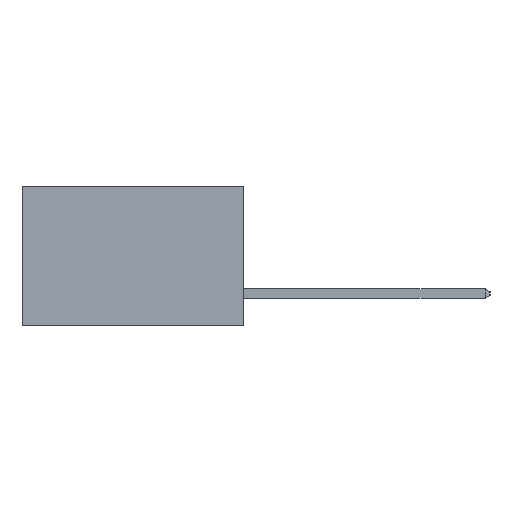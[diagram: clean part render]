
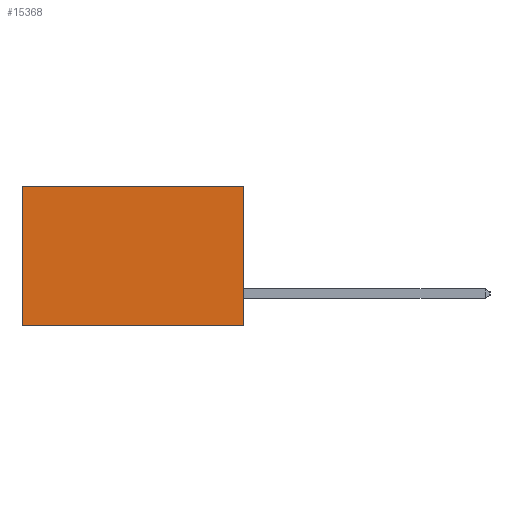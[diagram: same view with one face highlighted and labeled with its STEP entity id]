
A CAD part, left-side view. The second image highlights one B-rep face of the part: STEP entity #15368.
In plain terms, the highlighted planar face has unit normal (-1, 0, 0).
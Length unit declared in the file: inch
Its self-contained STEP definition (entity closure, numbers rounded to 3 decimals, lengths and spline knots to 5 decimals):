
#31 = VECTOR ( 'NONE', #7765, 39.37008 ) ;
#1726 = VECTOR ( 'NONE', #19805, 39.37008 ) ;
#2255 = VECTOR ( 'NONE', #12954, 39.37008 ) ;
#2284 = FACE_OUTER_BOUND ( 'NONE', #19009, .T. ) ;
#2792 = CARTESIAN_POINT ( 'NONE',  ( 0.277, 0.59, 0. ) ) ;
#2856 = EDGE_CURVE ( 'NONE', #18014, #8481, #8822, .T. ) ;
#4262 = LINE ( 'NONE', #10218, #20823 ) ;
#4377 = DIRECTION ( 'NONE',  ( 1., 0., 0. ) ) ;
#5814 = ORIENTED_EDGE ( 'NONE', *, *, #16967, .F. ) ;
#6081 = LINE ( 'NONE', #8632, #1726 ) ;
#7255 = CARTESIAN_POINT ( 'NONE',  ( 0.277, 0.59, -0.37 ) ) ;
#7581 = CARTESIAN_POINT ( 'NONE',  ( 0.277, 0., -0.37 ) ) ;
#7765 = DIRECTION ( 'NONE',  ( 0., 1., 0. ) ) ;
#8481 = VERTEX_POINT ( 'NONE', #7255 ) ;
#8632 = CARTESIAN_POINT ( 'NONE',  ( 0.277, 0., 0. ) ) ;
#8822 = LINE ( 'NONE', #17633, #31 ) ;
#9322 = VERTEX_POINT ( 'NONE', #2792 ) ;
#9854 = ORIENTED_EDGE ( 'NONE', *, *, #11756, .T. ) ;
#10218 = CARTESIAN_POINT ( 'NONE',  ( 0.277, 0., -0.37 ) ) ;
#11756 = EDGE_CURVE ( 'NONE', #9322, #8481, #15710, .T. ) ;
#12264 = AXIS2_PLACEMENT_3D ( 'NONE', #7581, #4377, #15701 ) ;
#12954 = DIRECTION ( 'NONE',  ( 0., 0., -1. ) ) ;
#13181 = CARTESIAN_POINT ( 'NONE',  ( 0.277, 0., -0.37 ) ) ;
#13471 = DIRECTION ( 'NONE',  ( 0., 0., -1. ) ) ;
#14090 = PLANE ( 'NONE',  #12264 ) ;
#14883 = VERTEX_POINT ( 'NONE', #19246 ) ;
#15368 = ADVANCED_FACE ( 'NONE', ( #2284 ), #14090, .F. ) ;
#15701 = DIRECTION ( 'NONE',  ( 0., 0., -1. ) ) ;
#15710 = LINE ( 'NONE', #20844, #2255 ) ;
#15923 = ORIENTED_EDGE ( 'NONE', *, *, #2856, .F. ) ;
#16291 = EDGE_CURVE ( 'NONE', #14883, #9322, #6081, .T. ) ;
#16967 = EDGE_CURVE ( 'NONE', #14883, #18014, #4262, .T. ) ;
#17633 = CARTESIAN_POINT ( 'NONE',  ( 0.277, 0., -0.37 ) ) ;
#18014 = VERTEX_POINT ( 'NONE', #13181 ) ;
#18469 = ORIENTED_EDGE ( 'NONE', *, *, #16291, .T. ) ;
#19009 = EDGE_LOOP ( 'NONE', ( #9854, #15923, #5814, #18469 ) ) ;
#19246 = CARTESIAN_POINT ( 'NONE',  ( 0.277, 0., 0. ) ) ;
#19805 = DIRECTION ( 'NONE',  ( 0., 1., 0. ) ) ;
#20823 = VECTOR ( 'NONE', #13471, 39.37008 ) ;
#20844 = CARTESIAN_POINT ( 'NONE',  ( 0.277, 0.59, -0.37 ) ) ;
